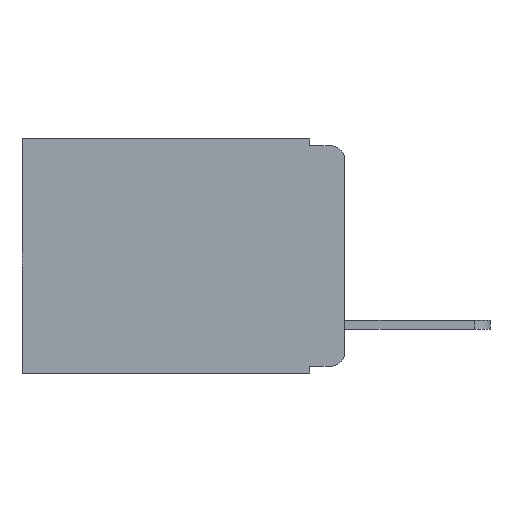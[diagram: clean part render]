
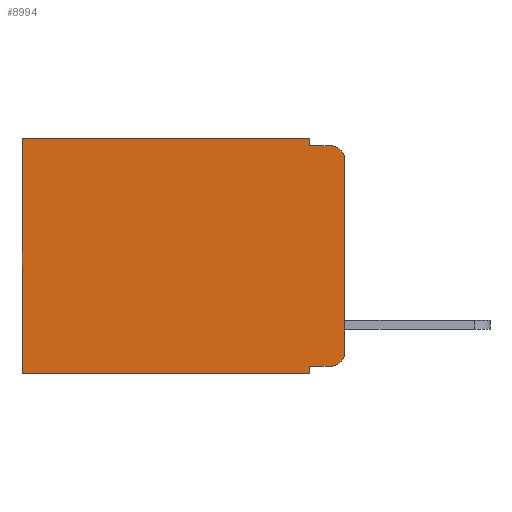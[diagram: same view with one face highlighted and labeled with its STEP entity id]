
A CAD part, left-side view. The second image highlights one B-rep face of the part: STEP entity #8994.
In plain terms, the highlighted planar face has unit normal (-1, 0, 0).
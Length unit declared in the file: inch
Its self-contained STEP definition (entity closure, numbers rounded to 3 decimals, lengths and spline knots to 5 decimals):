
#117 = VECTOR ( 'NONE', #17205, 39.37008 ) ;
#125 = VERTEX_POINT ( 'NONE', #5821 ) ;
#578 = CARTESIAN_POINT ( 'NONE',  ( 0.298, 0.051, -0.333 ) ) ;
#1165 = VERTEX_POINT ( 'NONE', #7566 ) ;
#1239 = LINE ( 'NONE', #17794, #15290 ) ;
#1273 = CARTESIAN_POINT ( 'NONE',  ( 0.298, 0., 0. ) ) ;
#1822 = VECTOR ( 'NONE', #18661, 39.37008 ) ;
#1939 = VECTOR ( 'NONE', #18302, 39.37008 ) ;
#2004 = CARTESIAN_POINT ( 'NONE',  ( 0.298, 0.051, -0.343 ) ) ;
#2202 = EDGE_CURVE ( 'NONE', #125, #16548, #3995, .T. ) ;
#2412 = ORIENTED_EDGE ( 'NONE', *, *, #18281, .T. ) ;
#2925 = EDGE_CURVE ( 'NONE', #16226, #14922, #4897, .T. ) ;
#3371 = CARTESIAN_POINT ( 'NONE',  ( 0.298, 0.051, 0. ) ) ;
#3720 = AXIS2_PLACEMENT_3D ( 'NONE', #10226, #4419, #17387 ) ;
#3954 = LINE ( 'NONE', #16669, #1939 ) ;
#3995 = LINE ( 'NONE', #10326, #17914 ) ;
#4419 = DIRECTION ( 'NONE',  ( 1., 0., 0. ) ) ;
#4544 = EDGE_CURVE ( 'NONE', #11878, #1165, #5908, .T. ) ;
#4897 = LINE ( 'NONE', #14241, #8320 ) ;
#5148 = CIRCLE ( 'NONE', #10713, 0.02 ) ;
#5303 = CARTESIAN_POINT ( 'NONE',  ( 0.298, 0.051, -0.01 ) ) ;
#5821 = CARTESIAN_POINT ( 'NONE',  ( 0.298, 0.473, 0. ) ) ;
#5908 = LINE ( 'NONE', #5303, #1822 ) ;
#6029 = CARTESIAN_POINT ( 'NONE',  ( 0.298, 0., -0.03 ) ) ;
#6340 = CARTESIAN_POINT ( 'NONE',  ( 0.298, 0.051, 0. ) ) ;
#7300 = DIRECTION ( 'NONE',  ( 0., 0., -1. ) ) ;
#7566 = CARTESIAN_POINT ( 'NONE',  ( 0.298, 0.02, -0.01 ) ) ;
#7612 = ORIENTED_EDGE ( 'NONE', *, *, #2925, .F. ) ;
#8320 = VECTOR ( 'NONE', #8369, 39.37008 ) ;
#8333 = CARTESIAN_POINT ( 'NONE',  ( 0.298, 0., -0.313 ) ) ;
#8369 = DIRECTION ( 'NONE',  ( 0., 0., -1. ) ) ;
#8452 = VERTEX_POINT ( 'NONE', #8333 ) ;
#8762 = DIRECTION ( 'NONE',  ( -1., 0., 0. ) ) ;
#8994 = ADVANCED_FACE ( 'NONE', ( #9836 ), #16181, .F. ) ;
#9125 = DIRECTION ( 'NONE',  ( 0., 0., -1. ) ) ;
#9406 = LINE ( 'NONE', #14245, #18255 ) ;
#9809 = CIRCLE ( 'NONE', #12832, 0.02 ) ;
#9824 = EDGE_CURVE ( 'NONE', #16691, #8452, #9809, .T. ) ;
#9836 = FACE_OUTER_BOUND ( 'NONE', #13947, .T. ) ;
#9919 = EDGE_CURVE ( 'NONE', #14922, #16548, #1239, .T. ) ;
#10226 = CARTESIAN_POINT ( 'NONE',  ( 0.298, 0., 0. ) ) ;
#10229 = CARTESIAN_POINT ( 'NONE',  ( 0.298, 0.02, -0.333 ) ) ;
#10326 = CARTESIAN_POINT ( 'NONE',  ( 0.298, 0.473, 0. ) ) ;
#10713 = AXIS2_PLACEMENT_3D ( 'NONE', #14644, #8762, #7300 ) ;
#10783 = LINE ( 'NONE', #1273, #117 ) ;
#11296 = ORIENTED_EDGE ( 'NONE', *, *, #9919, .F. ) ;
#11878 = VERTEX_POINT ( 'NONE', #12702 ) ;
#12088 = DIRECTION ( 'NONE',  ( 0., 1., 0. ) ) ;
#12702 = CARTESIAN_POINT ( 'NONE',  ( 0.298, 0.051, -0.01 ) ) ;
#12832 = AXIS2_PLACEMENT_3D ( 'NONE', #14866, #16353, #9125 ) ;
#13545 = CARTESIAN_POINT ( 'NONE',  ( 0.298, 0.473, -0.343 ) ) ;
#13757 = EDGE_CURVE ( 'NONE', #16226, #16691, #3954, .T. ) ;
#13934 = LINE ( 'NONE', #6340, #18725 ) ;
#13947 = EDGE_LOOP ( 'NONE', ( #17673, #18699, #14835, #14310, #2412, #18475, #11296, #7612, #17022, #17981 ) ) ;
#14241 = CARTESIAN_POINT ( 'NONE',  ( 0.298, 0.051, 0. ) ) ;
#14245 = CARTESIAN_POINT ( 'NONE',  ( 0.298, 0., 0. ) ) ;
#14304 = EDGE_CURVE ( 'NONE', #17990, #11878, #13934, .T. ) ;
#14310 = ORIENTED_EDGE ( 'NONE', *, *, #14304, .F. ) ;
#14508 = DIRECTION ( 'NONE',  ( 0., 0., -1. ) ) ;
#14644 = CARTESIAN_POINT ( 'NONE',  ( 0.298, 0.02, -0.03 ) ) ;
#14650 = EDGE_CURVE ( 'NONE', #16050, #8452, #9406, .T. ) ;
#14835 = ORIENTED_EDGE ( 'NONE', *, *, #4544, .F. ) ;
#14866 = CARTESIAN_POINT ( 'NONE',  ( 0.298, 0.02, -0.313 ) ) ;
#14922 = VERTEX_POINT ( 'NONE', #2004 ) ;
#15045 = DIRECTION ( 'NONE',  ( 0., 0., -1. ) ) ;
#15290 = VECTOR ( 'NONE', #12088, 39.37008 ) ;
#16050 = VERTEX_POINT ( 'NONE', #6029 ) ;
#16181 = PLANE ( 'NONE',  #3720 ) ;
#16226 = VERTEX_POINT ( 'NONE', #578 ) ;
#16353 = DIRECTION ( 'NONE',  ( -1., 0., 0. ) ) ;
#16548 = VERTEX_POINT ( 'NONE', #13545 ) ;
#16637 = EDGE_CURVE ( 'NONE', #16050, #1165, #5148, .T. ) ;
#16669 = CARTESIAN_POINT ( 'NONE',  ( 0.298, 0.051, -0.333 ) ) ;
#16691 = VERTEX_POINT ( 'NONE', #10229 ) ;
#17022 = ORIENTED_EDGE ( 'NONE', *, *, #13757, .T. ) ;
#17205 = DIRECTION ( 'NONE',  ( 0., 1., 0. ) ) ;
#17387 = DIRECTION ( 'NONE',  ( 0., 0., -1. ) ) ;
#17561 = DIRECTION ( 'NONE',  ( 0., 0., -1. ) ) ;
#17673 = ORIENTED_EDGE ( 'NONE', *, *, #14650, .F. ) ;
#17794 = CARTESIAN_POINT ( 'NONE',  ( 0.298, 0., -0.343 ) ) ;
#17914 = VECTOR ( 'NONE', #17561, 39.37008 ) ;
#17981 = ORIENTED_EDGE ( 'NONE', *, *, #9824, .T. ) ;
#17990 = VERTEX_POINT ( 'NONE', #3371 ) ;
#18255 = VECTOR ( 'NONE', #14508, 39.37008 ) ;
#18281 = EDGE_CURVE ( 'NONE', #17990, #125, #10783, .T. ) ;
#18302 = DIRECTION ( 'NONE',  ( 0., -1., 0. ) ) ;
#18475 = ORIENTED_EDGE ( 'NONE', *, *, #2202, .T. ) ;
#18661 = DIRECTION ( 'NONE',  ( 0., -1., 0. ) ) ;
#18699 = ORIENTED_EDGE ( 'NONE', *, *, #16637, .T. ) ;
#18725 = VECTOR ( 'NONE', #15045, 39.37008 ) ;
